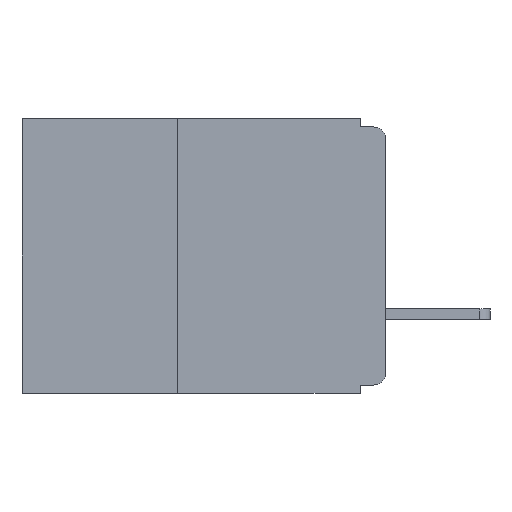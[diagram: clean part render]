
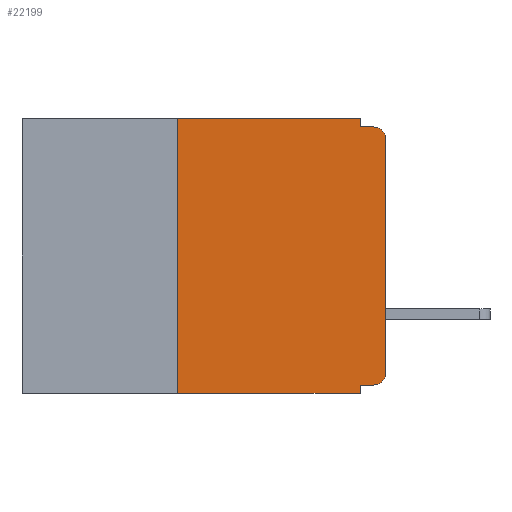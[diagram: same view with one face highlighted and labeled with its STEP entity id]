
A CAD part, left-side view. The second image highlights one B-rep face of the part: STEP entity #22199.
In plain terms, the highlighted planar face has unit normal (-1, 0, 0).
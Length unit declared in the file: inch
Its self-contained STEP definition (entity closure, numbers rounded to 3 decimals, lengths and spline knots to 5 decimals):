
#43 = DIRECTION ( 'NONE',  ( -1., 0., 0. ) ) ;
#916 = CARTESIAN_POINT ( 'NONE',  ( 0., 0., -0.025 ) ) ;
#976 = VECTOR ( 'NONE', #18629, 39.37008 ) ;
#984 = EDGE_CURVE ( 'NONE', #15900, #22548, #8182, .T. ) ;
#1127 = VERTEX_POINT ( 'NONE', #916 ) ;
#1585 = DIRECTION ( 'NONE',  ( 0., 0., -1. ) ) ;
#1830 = CARTESIAN_POINT ( 'NONE',  ( 0., 0., 0. ) ) ;
#1841 = CARTESIAN_POINT ( 'NONE',  ( 0., 0., -0.01 ) ) ;
#2034 = EDGE_CURVE ( 'NONE', #23741, #8347, #2600, .T. ) ;
#2311 = CARTESIAN_POINT ( 'NONE',  ( 0., 0.25, -0.33 ) ) ;
#2600 = LINE ( 'NONE', #8877, #13291 ) ;
#2623 = CARTESIAN_POINT ( 'NONE',  ( 0., 0.031, -0.32 ) ) ;
#2782 = VECTOR ( 'NONE', #8875, 39.37008 ) ;
#3293 = PLANE ( 'NONE',  #10914 ) ;
#3556 = VERTEX_POINT ( 'NONE', #14953 ) ;
#3790 = ORIENTED_EDGE ( 'NONE', *, *, #13915, .T. ) ;
#4323 = CARTESIAN_POINT ( 'NONE',  ( 0., 0.031, 0. ) ) ;
#4446 = VERTEX_POINT ( 'NONE', #13784 ) ;
#4493 = CIRCLE ( 'NONE', #22681, 0.015 ) ;
#4569 = VECTOR ( 'NONE', #9336, 39.37008 ) ;
#4780 = VERTEX_POINT ( 'NONE', #5975 ) ;
#5136 = LINE ( 'NONE', #1841, #4569 ) ;
#5143 = DIRECTION ( 'NONE',  ( 0., 0., -1. ) ) ;
#5410 = CARTESIAN_POINT ( 'NONE',  ( 0., 0.031, -0.33 ) ) ;
#5975 = CARTESIAN_POINT ( 'NONE',  ( 0., 0., -0.305 ) ) ;
#6012 = LINE ( 'NONE', #2311, #15607 ) ;
#6529 = EDGE_CURVE ( 'NONE', #4780, #1127, #22931, .T. ) ;
#6655 = VERTEX_POINT ( 'NONE', #17412 ) ;
#7119 = EDGE_CURVE ( 'NONE', #1127, #4446, #12469, .T. ) ;
#7423 = ORIENTED_EDGE ( 'NONE', *, *, #984, .F. ) ;
#7589 = VECTOR ( 'NONE', #23302, 39.37008 ) ;
#8182 = LINE ( 'NONE', #10057, #7589 ) ;
#8347 = VERTEX_POINT ( 'NONE', #5410 ) ;
#8475 = FACE_OUTER_BOUND ( 'NONE', #8846, .T. ) ;
#8846 = EDGE_LOOP ( 'NONE', ( #14500, #20436, #22302, #11338, #7423, #12009, #24198, #20413, #16048, #3790 ) ) ;
#8875 = DIRECTION ( 'NONE',  ( 0., 1., 0. ) ) ;
#8877 = CARTESIAN_POINT ( 'NONE',  ( 0., 0.031, -0.33 ) ) ;
#9336 = DIRECTION ( 'NONE',  ( 0., -1., 0. ) ) ;
#10057 = CARTESIAN_POINT ( 'NONE',  ( 0., 0.437, 0. ) ) ;
#10142 = EDGE_CURVE ( 'NONE', #3556, #4446, #5136, .T. ) ;
#10609 = EDGE_CURVE ( 'NONE', #19926, #23741, #17935, .T. ) ;
#10718 = CARTESIAN_POINT ( 'NONE',  ( 0., 0.437, 0. ) ) ;
#10914 = AXIS2_PLACEMENT_3D ( 'NONE', #10718, #16588, #5143 ) ;
#11314 = CARTESIAN_POINT ( 'NONE',  ( 0., 0.015, -0.025 ) ) ;
#11338 = ORIENTED_EDGE ( 'NONE', *, *, #14547, .F. ) ;
#12009 = ORIENTED_EDGE ( 'NONE', *, *, #23643, .F. ) ;
#12469 = CIRCLE ( 'NONE', #16677, 0.015 ) ;
#12913 = DIRECTION ( 'NONE',  ( -1., 0., 0. ) ) ;
#13186 = DIRECTION ( 'NONE',  ( 0., 0., 1. ) ) ;
#13243 = DIRECTION ( 'NONE',  ( 0., 0., -1. ) ) ;
#13291 = VECTOR ( 'NONE', #19019, 39.37008 ) ;
#13784 = CARTESIAN_POINT ( 'NONE',  ( 0., 0.015, -0.01 ) ) ;
#13915 = EDGE_CURVE ( 'NONE', #19926, #4780, #4493, .T. ) ;
#14500 = ORIENTED_EDGE ( 'NONE', *, *, #6529, .T. ) ;
#14547 = EDGE_CURVE ( 'NONE', #22548, #3556, #16089, .T. ) ;
#14953 = CARTESIAN_POINT ( 'NONE',  ( 0., 0.031, -0.01 ) ) ;
#15607 = VECTOR ( 'NONE', #17487, 39.37008 ) ;
#15900 = VERTEX_POINT ( 'NONE', #24426 ) ;
#16048 = ORIENTED_EDGE ( 'NONE', *, *, #10609, .F. ) ;
#16089 = LINE ( 'NONE', #16738, #976 ) ;
#16588 = DIRECTION ( 'NONE',  ( 1., 0., 0. ) ) ;
#16677 = AXIS2_PLACEMENT_3D ( 'NONE', #11314, #43, #13243 ) ;
#16738 = CARTESIAN_POINT ( 'NONE',  ( 0., 0.031, 0. ) ) ;
#17258 = VECTOR ( 'NONE', #13186, 39.37008 ) ;
#17412 = CARTESIAN_POINT ( 'NONE',  ( 0., 0.25, -0.33 ) ) ;
#17487 = DIRECTION ( 'NONE',  ( 0., 0., 1. ) ) ;
#17560 = DIRECTION ( 'NONE',  ( 0., -1., 0. ) ) ;
#17935 = LINE ( 'NONE', #20242, #2782 ) ;
#18629 = DIRECTION ( 'NONE',  ( 0., 0., -1. ) ) ;
#19019 = DIRECTION ( 'NONE',  ( 0., 0., -1. ) ) ;
#19451 = VECTOR ( 'NONE', #17560, 39.37008 ) ;
#19926 = VERTEX_POINT ( 'NONE', #20143 ) ;
#20143 = CARTESIAN_POINT ( 'NONE',  ( 0., 0.015, -0.32 ) ) ;
#20242 = CARTESIAN_POINT ( 'NONE',  ( 0., 0., -0.32 ) ) ;
#20413 = ORIENTED_EDGE ( 'NONE', *, *, #2034, .F. ) ;
#20436 = ORIENTED_EDGE ( 'NONE', *, *, #7119, .T. ) ;
#22199 = ADVANCED_FACE ( 'NONE', ( #8475 ), #3293, .F. ) ;
#22302 = ORIENTED_EDGE ( 'NONE', *, *, #10142, .F. ) ;
#22548 = VERTEX_POINT ( 'NONE', #4323 ) ;
#22681 = AXIS2_PLACEMENT_3D ( 'NONE', #24328, #12913, #1585 ) ;
#22931 = LINE ( 'NONE', #1830, #17258 ) ;
#23302 = DIRECTION ( 'NONE',  ( 0., -1., 0. ) ) ;
#23317 = CARTESIAN_POINT ( 'NONE',  ( 0., 0.437, -0.33 ) ) ;
#23643 = EDGE_CURVE ( 'NONE', #6655, #15900, #6012, .T. ) ;
#23691 = EDGE_CURVE ( 'NONE', #6655, #8347, #24520, .T. ) ;
#23741 = VERTEX_POINT ( 'NONE', #2623 ) ;
#24198 = ORIENTED_EDGE ( 'NONE', *, *, #23691, .T. ) ;
#24328 = CARTESIAN_POINT ( 'NONE',  ( 0., 0.015, -0.305 ) ) ;
#24426 = CARTESIAN_POINT ( 'NONE',  ( 0., 0.25, 0. ) ) ;
#24520 = LINE ( 'NONE', #23317, #19451 ) ;
